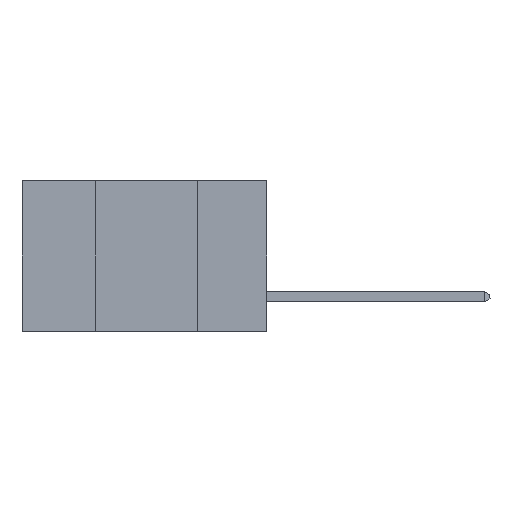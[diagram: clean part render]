
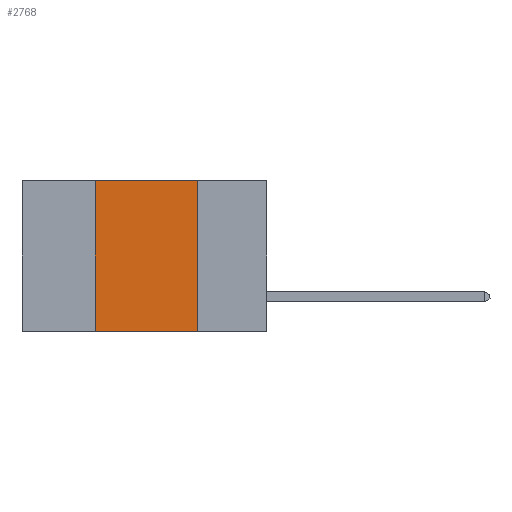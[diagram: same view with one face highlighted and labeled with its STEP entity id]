
A CAD part, left-side view. The second image highlights one B-rep face of the part: STEP entity #2768.
In plain terms, the highlighted planar face has unit normal (-1, 0, 0).
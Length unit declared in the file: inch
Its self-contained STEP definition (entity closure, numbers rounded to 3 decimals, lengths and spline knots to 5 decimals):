
#379 = CARTESIAN_POINT ( 'NONE',  ( 0., 0.6, 0. ) ) ;
#934 = DIRECTION ( 'NONE',  ( 0., 0., -1. ) ) ;
#1066 = PLANE ( 'NONE',  #13265 ) ;
#1304 = CARTESIAN_POINT ( 'NONE',  ( 0., 0.6, -0.37 ) ) ;
#1497 = CARTESIAN_POINT ( 'NONE',  ( 0., 0.17, 0. ) ) ;
#1667 = VECTOR ( 'NONE', #934, 39.37008 ) ;
#1739 = FACE_OUTER_BOUND ( 'NONE', #9916, .T. ) ;
#2768 = ADVANCED_FACE ( 'NONE', ( #1739 ), #1066, .F. ) ;
#4075 = EDGE_CURVE ( 'NONE', #10123, #10221, #8776, .T. ) ;
#4222 = EDGE_CURVE ( 'NONE', #4247, #10221, #4882, .T. ) ;
#4247 = VERTEX_POINT ( 'NONE', #9661 ) ;
#4253 = EDGE_CURVE ( 'NONE', #10123, #10588, #12691, .T. ) ;
#4880 = CARTESIAN_POINT ( 'NONE',  ( 0., 0.42, 0. ) ) ;
#4882 = LINE ( 'NONE', #1497, #1667 ) ;
#5619 = CARTESIAN_POINT ( 'NONE',  ( 0., 0.42, 0. ) ) ;
#6137 = DIRECTION ( 'NONE',  ( 0., -1., 0. ) ) ;
#7295 = EDGE_CURVE ( 'NONE', #10588, #4247, #13330, .T. ) ;
#8776 = LINE ( 'NONE', #1304, #13486 ) ;
#9042 = DIRECTION ( 'NONE',  ( 1., 0., 0. ) ) ;
#9661 = CARTESIAN_POINT ( 'NONE',  ( 0., 0.17, 0. ) ) ;
#9712 = VECTOR ( 'NONE', #11713, 39.37008 ) ;
#9830 = CARTESIAN_POINT ( 'NONE',  ( 0., 0.6, 0. ) ) ;
#9916 = EDGE_LOOP ( 'NONE', ( #13011, #13057, #12742, #12689 ) ) ;
#10052 = DIRECTION ( 'NONE',  ( 0., 0., -1. ) ) ;
#10123 = VERTEX_POINT ( 'NONE', #12527 ) ;
#10221 = VERTEX_POINT ( 'NONE', #13592 ) ;
#10588 = VERTEX_POINT ( 'NONE', #4880 ) ;
#10671 = VECTOR ( 'NONE', #6137, 39.37008 ) ;
#11282 = DIRECTION ( 'NONE',  ( 0., -1., 0. ) ) ;
#11713 = DIRECTION ( 'NONE',  ( 0., 0., 1. ) ) ;
#12527 = CARTESIAN_POINT ( 'NONE',  ( 0., 0.42, -0.37 ) ) ;
#12689 = ORIENTED_EDGE ( 'NONE', *, *, #4075, .T. ) ;
#12691 = LINE ( 'NONE', #5619, #9712 ) ;
#12742 = ORIENTED_EDGE ( 'NONE', *, *, #4253, .F. ) ;
#13011 = ORIENTED_EDGE ( 'NONE', *, *, #4222, .F. ) ;
#13057 = ORIENTED_EDGE ( 'NONE', *, *, #7295, .F. ) ;
#13265 = AXIS2_PLACEMENT_3D ( 'NONE', #9830, #9042, #10052 ) ;
#13330 = LINE ( 'NONE', #379, #10671 ) ;
#13486 = VECTOR ( 'NONE', #11282, 39.37008 ) ;
#13592 = CARTESIAN_POINT ( 'NONE',  ( 0., 0.17, -0.37 ) ) ;
